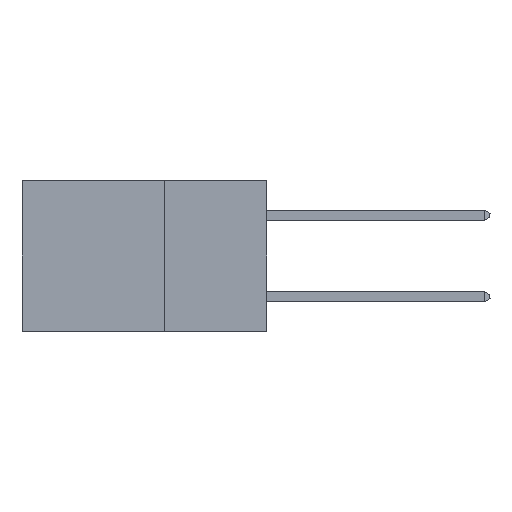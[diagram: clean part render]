
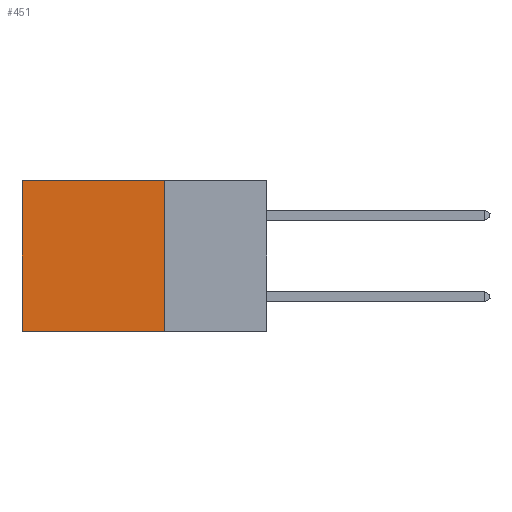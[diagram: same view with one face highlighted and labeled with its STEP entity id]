
A CAD part, left-side view. The second image highlights one B-rep face of the part: STEP entity #451.
In plain terms, the highlighted planar face has unit normal (-1, 0, 0).
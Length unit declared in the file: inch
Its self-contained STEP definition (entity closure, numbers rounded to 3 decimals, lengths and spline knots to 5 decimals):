
#451 = ADVANCED_FACE ( 'NONE', ( #15064 ), #11676, .F. ) ;
#974 = CARTESIAN_POINT ( 'NONE',  ( 0.2875, 0.25, -0.37 ) ) ;
#1307 = VECTOR ( 'NONE', #18509, 39.37008 ) ;
#2562 = CARTESIAN_POINT ( 'NONE',  ( 0.2875, 0.25, 0. ) ) ;
#2878 = CARTESIAN_POINT ( 'NONE',  ( 0.2875, 0.25, 0. ) ) ;
#3142 = LINE ( 'NONE', #19476, #16416 ) ;
#4507 = CARTESIAN_POINT ( 'NONE',  ( 0.2875, 0.25, 0. ) ) ;
#4555 = LINE ( 'NONE', #974, #21914 ) ;
#4713 = EDGE_LOOP ( 'NONE', ( #17043, #13176, #10081, #16028 ) ) ;
#7372 = EDGE_CURVE ( 'NONE', #21877, #13921, #10276, .T. ) ;
#7848 = LINE ( 'NONE', #10189, #8638 ) ;
#8638 = VECTOR ( 'NONE', #20548, 39.37008 ) ;
#10081 = ORIENTED_EDGE ( 'NONE', *, *, #17029, .F. ) ;
#10189 = CARTESIAN_POINT ( 'NONE',  ( 0.2875, 0.6, 0. ) ) ;
#10276 = LINE ( 'NONE', #2878, #1307 ) ;
#11309 = DIRECTION ( 'NONE',  ( 0., 1., 0. ) ) ;
#11676 = PLANE ( 'NONE',  #20437 ) ;
#13176 = ORIENTED_EDGE ( 'NONE', *, *, #15266, .F. ) ;
#13921 = VERTEX_POINT ( 'NONE', #15213 ) ;
#14764 = EDGE_CURVE ( 'NONE', #13921, #22227, #7848, .T. ) ;
#15064 = FACE_OUTER_BOUND ( 'NONE', #4713, .T. ) ;
#15213 = CARTESIAN_POINT ( 'NONE',  ( 0.2875, 0.6, 0. ) ) ;
#15266 = EDGE_CURVE ( 'NONE', #19342, #22227, #4555, .T. ) ;
#15968 = CARTESIAN_POINT ( 'NONE',  ( 0.2875, 0.25, -0.37 ) ) ;
#16028 = ORIENTED_EDGE ( 'NONE', *, *, #7372, .T. ) ;
#16416 = VECTOR ( 'NONE', #16900, 39.37008 ) ;
#16900 = DIRECTION ( 'NONE',  ( 0., 0., -1. ) ) ;
#17029 = EDGE_CURVE ( 'NONE', #21877, #19342, #3142, .T. ) ;
#17043 = ORIENTED_EDGE ( 'NONE', *, *, #14764, .T. ) ;
#18509 = DIRECTION ( 'NONE',  ( 0., 1., 0. ) ) ;
#19342 = VERTEX_POINT ( 'NONE', #15968 ) ;
#19476 = CARTESIAN_POINT ( 'NONE',  ( 0.2875, 0.25, 0. ) ) ;
#20437 = AXIS2_PLACEMENT_3D ( 'NONE', #4507, #20881, #21110 ) ;
#20548 = DIRECTION ( 'NONE',  ( 0., 0., -1. ) ) ;
#20690 = CARTESIAN_POINT ( 'NONE',  ( 0.2875, 0.6, -0.37 ) ) ;
#20881 = DIRECTION ( 'NONE',  ( 1., 0., 0. ) ) ;
#21110 = DIRECTION ( 'NONE',  ( 0., 0., -1. ) ) ;
#21877 = VERTEX_POINT ( 'NONE', #2562 ) ;
#21914 = VECTOR ( 'NONE', #11309, 39.37008 ) ;
#22227 = VERTEX_POINT ( 'NONE', #20690 ) ;
